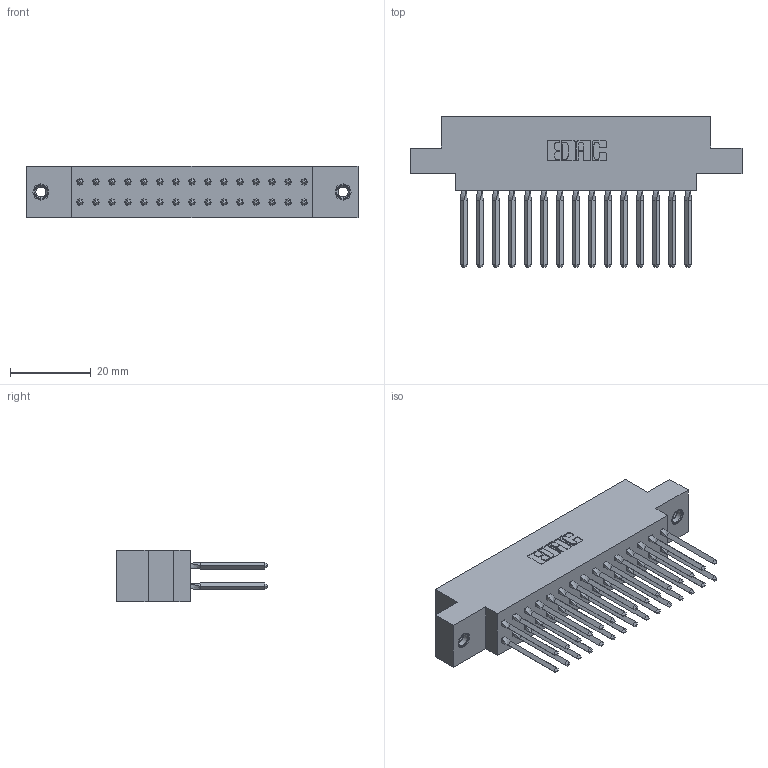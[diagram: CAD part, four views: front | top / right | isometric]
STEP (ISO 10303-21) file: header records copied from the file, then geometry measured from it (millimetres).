
FILE_DESCRIPTION (( 'STEP AP203' ), '1' );
FILE_NAME ('317-030-540-807.STEP', '2020-02-27T20:21:53', ( '' ), ( '' ), 'SwSTEP 2.0', 'SolidWorks 2016', '' );
FILE_SCHEMA (( 'CONFIG_CONTROL_DESIGN' ));
Length unit declared in the file: inch
Products named in the file (4): 317 Part_.156 Dia - TI; 345-250-001_345-250-005-103; 317-030-540-807; 317-290-001_540
Assembly tree (33 placements, depth 2):
  317-030-540-807
    317 Part_.156 Dia - TI
    317-290-001_540  x30
    345-250-001_345-250-005-103  x2
Bounding box: 82.14 x 37.34 x 12.7 mm (x, y, z)
Volume: 12859.8 mm3; surface area: 18189.7 mm2
Topology: 33 solids, 33 shells, 2832 faces, 7821 edges, 5036 vertices
Faces by surface type: plane 2280, cylinder 416, bspline 120, cone 12, torus 4
Entity records: 26635 total; most frequent: CARTESIAN_POINT 5030, ORIENTED_EDGE 4522, DIRECTION 3817, EDGE_CURVE 2261, VECTOR 1985, LINE 1985, VERTEX_POINT 1497, AXIS2_PLACEMENT_3D 916
